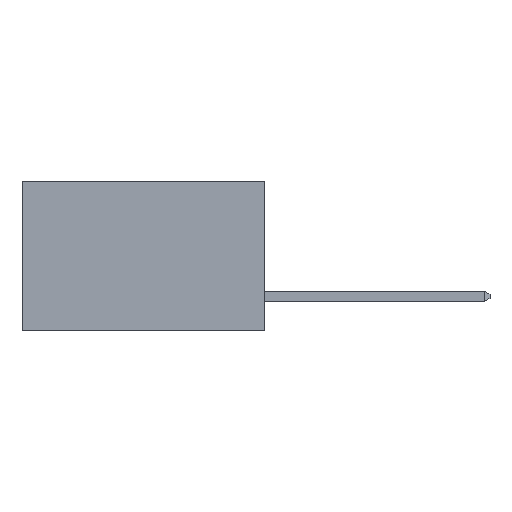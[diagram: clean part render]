
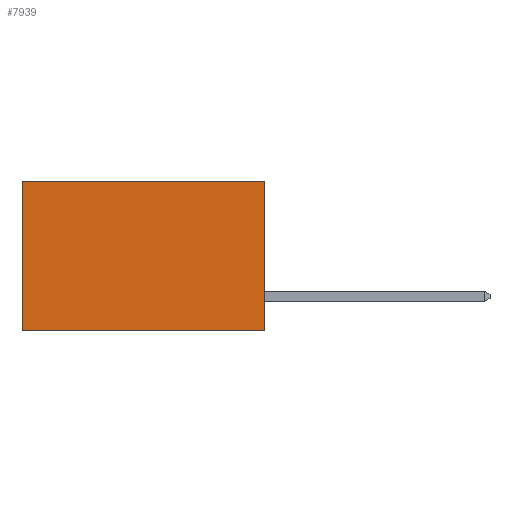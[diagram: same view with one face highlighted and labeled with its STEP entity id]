
A CAD part, left-side view. The second image highlights one B-rep face of the part: STEP entity #7939.
In plain terms, the highlighted planar face has unit normal (-1, 0, 0).
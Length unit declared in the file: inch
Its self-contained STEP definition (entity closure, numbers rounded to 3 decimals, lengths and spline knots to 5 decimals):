
#354 = ORIENTED_EDGE ( 'NONE', *, *, #5360, .F. ) ;
#554 = EDGE_CURVE ( 'NONE', #3832, #2495, #8872, .T. ) ;
#1060 = CARTESIAN_POINT ( 'NONE',  ( 0.2615, 0., -0.37 ) ) ;
#1203 = CARTESIAN_POINT ( 'NONE',  ( 0.2615, 0., -0.37 ) ) ;
#1269 = EDGE_CURVE ( 'NONE', #2495, #8969, #3959, .T. ) ;
#1470 = ORIENTED_EDGE ( 'NONE', *, *, #1269, .T. ) ;
#1496 = VERTEX_POINT ( 'NONE', #1203 ) ;
#1892 = CARTESIAN_POINT ( 'NONE',  ( 0.2615, 0.6, 0. ) ) ;
#2114 = CARTESIAN_POINT ( 'NONE',  ( 0.2615, 0., -0.37 ) ) ;
#2229 = VECTOR ( 'NONE', #4697, 39.37008 ) ;
#2495 = VERTEX_POINT ( 'NONE', #1892 ) ;
#2596 = DIRECTION ( 'NONE',  ( 1., 0., 0. ) ) ;
#2827 = LINE ( 'NONE', #2114, #5059 ) ;
#3095 = VECTOR ( 'NONE', #3672, 39.37008 ) ;
#3672 = DIRECTION ( 'NONE',  ( 0., 1., 0. ) ) ;
#3714 = ORIENTED_EDGE ( 'NONE', *, *, #8222, .F. ) ;
#3777 = LINE ( 'NONE', #4728, #2229 ) ;
#3832 = VERTEX_POINT ( 'NONE', #7366 ) ;
#3959 = LINE ( 'NONE', #5920, #5726 ) ;
#4697 = DIRECTION ( 'NONE',  ( 0., 0., -1. ) ) ;
#4728 = CARTESIAN_POINT ( 'NONE',  ( 0.2615, 0., -0.37 ) ) ;
#4945 = EDGE_LOOP ( 'NONE', ( #1470, #3714, #354, #8467 ) ) ;
#4948 = FACE_OUTER_BOUND ( 'NONE', #4945, .T. ) ;
#5059 = VECTOR ( 'NONE', #6598, 39.37008 ) ;
#5360 = EDGE_CURVE ( 'NONE', #3832, #1496, #3777, .T. ) ;
#5559 = DIRECTION ( 'NONE',  ( 0., 0., -1. ) ) ;
#5726 = VECTOR ( 'NONE', #5559, 39.37008 ) ;
#5920 = CARTESIAN_POINT ( 'NONE',  ( 0.2615, 0.6, -0.37 ) ) ;
#6598 = DIRECTION ( 'NONE',  ( 0., 1., 0. ) ) ;
#7016 = PLANE ( 'NONE',  #8404 ) ;
#7366 = CARTESIAN_POINT ( 'NONE',  ( 0.2615, 0., 0. ) ) ;
#7450 = CARTESIAN_POINT ( 'NONE',  ( 0.2615, 0., 0. ) ) ;
#7762 = DIRECTION ( 'NONE',  ( 0., 0., -1. ) ) ;
#7939 = ADVANCED_FACE ( 'NONE', ( #4948 ), #7016, .F. ) ;
#8222 = EDGE_CURVE ( 'NONE', #1496, #8969, #2827, .T. ) ;
#8404 = AXIS2_PLACEMENT_3D ( 'NONE', #1060, #2596, #7762 ) ;
#8467 = ORIENTED_EDGE ( 'NONE', *, *, #554, .T. ) ;
#8694 = CARTESIAN_POINT ( 'NONE',  ( 0.2615, 0.6, -0.37 ) ) ;
#8872 = LINE ( 'NONE', #7450, #3095 ) ;
#8969 = VERTEX_POINT ( 'NONE', #8694 ) ;
